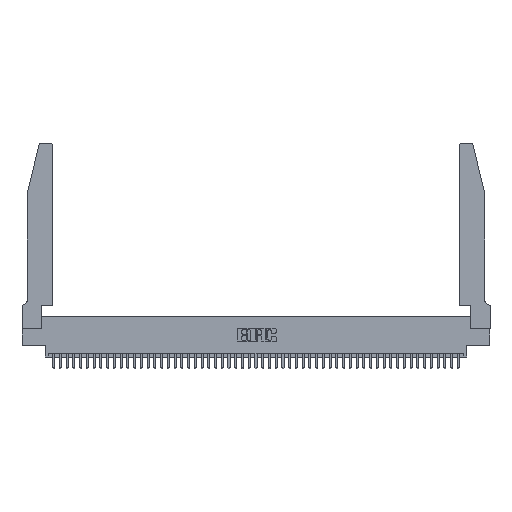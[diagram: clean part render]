
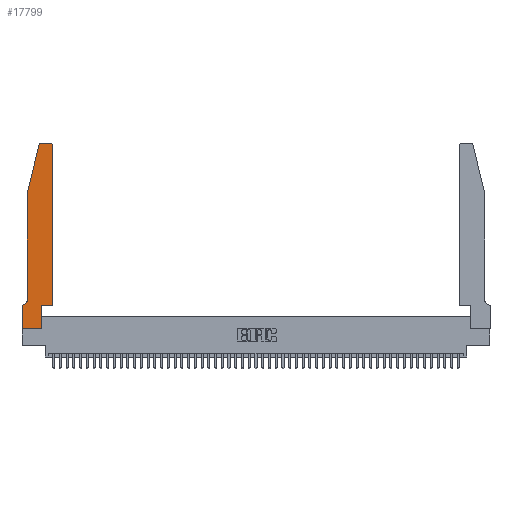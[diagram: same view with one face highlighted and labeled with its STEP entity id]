
A CAD part, top view. The second image highlights one B-rep face of the part: STEP entity #17799.
In plain terms, the highlighted planar face has unit normal (0, 0, 1).
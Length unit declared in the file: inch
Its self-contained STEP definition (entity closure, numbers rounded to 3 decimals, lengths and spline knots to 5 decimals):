
#931 = VERTEX_POINT ( 'NONE', #44905 ) ;
#1089 = LINE ( 'NONE', #2913, #20563 ) ;
#1990 = CARTESIAN_POINT ( 'NONE',  ( 0., 0., 0.37 ) ) ;
#2110 = EDGE_CURVE ( 'NONE', #21320, #24705, #28007, .T. ) ;
#2913 = CARTESIAN_POINT ( 'NONE',  ( 0., 0., 0.37 ) ) ;
#4332 = VECTOR ( 'NONE', #21773, 39.37008 ) ;
#4619 = CIRCLE ( 'NONE', #29182, 0.03 ) ;
#4855 = VECTOR ( 'NONE', #25329, 39.37008 ) ;
#6502 = CIRCLE ( 'NONE', #38145, 0.03 ) ;
#6902 = CARTESIAN_POINT ( 'NONE',  ( 0.4205, 2.72, 0.37 ) ) ;
#7082 = AXIS2_PLACEMENT_3D ( 'NONE', #7300, #34526, #11219 ) ;
#7300 = CARTESIAN_POINT ( 'NONE',  ( 0.0055, 0.42, 0.37 ) ) ;
#7564 = LINE ( 'NONE', #30500, #37380 ) ;
#8010 = VERTEX_POINT ( 'NONE', #41434 ) ;
#8220 = VERTEX_POINT ( 'NONE', #42438 ) ;
#9309 = FACE_OUTER_BOUND ( 'NONE', #49235, .T. ) ;
#10823 = DIRECTION ( 'NONE',  ( 1., 0., 0. ) ) ;
#11059 = VECTOR ( 'NONE', #26213, 39.37008 ) ;
#11179 = ORIENTED_EDGE ( 'NONE', *, *, #36745, .T. ) ;
#11219 = DIRECTION ( 'NONE',  ( -1., 0., 0. ) ) ;
#11917 = LINE ( 'NONE', #21364, #31407 ) ;
#11985 = EDGE_CURVE ( 'NONE', #36430, #46390, #40725, .T. ) ;
#12935 = CARTESIAN_POINT ( 'NONE',  ( 0., 0.35, 0.37 ) ) ;
#14453 = CARTESIAN_POINT ( 'NONE',  ( 0.4505, 0.35, 0.37 ) ) ;
#15032 = CARTESIAN_POINT ( 'NONE',  ( 0., 0., 0.37 ) ) ;
#15591 = VERTEX_POINT ( 'NONE', #47772 ) ;
#17471 = DIRECTION ( 'NONE',  ( 0., 1., 0. ) ) ;
#17622 = CARTESIAN_POINT ( 'NONE',  ( 0.0755, 2., 0.37 ) ) ;
#17799 = ADVANCED_FACE ( 'NONE', ( #9309 ), #46205, .T. ) ;
#17869 = CARTESIAN_POINT ( 'NONE',  ( 0.0755, 0.35, 0.37 ) ) ;
#18626 = VERTEX_POINT ( 'NONE', #50004 ) ;
#19388 = CARTESIAN_POINT ( 'NONE',  ( 0.284, 2.72, 0.37 ) ) ;
#20034 = VECTOR ( 'NONE', #36182, 39.37008 ) ;
#20265 = DIRECTION ( 'NONE',  ( 0., -1., 0. ) ) ;
#20518 = CARTESIAN_POINT ( 'NONE',  ( 0.4505, 0.35, 0.37 ) ) ;
#20535 = AXIS2_PLACEMENT_3D ( 'NONE', #49934, #50103, #49390 ) ;
#20563 = VECTOR ( 'NONE', #30157, 39.37008 ) ;
#21257 = ORIENTED_EDGE ( 'NONE', *, *, #28852, .T. ) ;
#21320 = VERTEX_POINT ( 'NONE', #12935 ) ;
#21356 = LINE ( 'NONE', #14453, #11059 ) ;
#21364 = CARTESIAN_POINT ( 'NONE',  ( 0.2865, 0.35, 0.37 ) ) ;
#21773 = DIRECTION ( 'NONE',  ( -1., 0., 0. ) ) ;
#22498 = ORIENTED_EDGE ( 'NONE', *, *, #32396, .T. ) ;
#22537 = LINE ( 'NONE', #40074, #41991 ) ;
#23283 = DIRECTION ( 'NONE',  ( 1., 0., 0. ) ) ;
#24360 = CARTESIAN_POINT ( 'NONE',  ( 0.0755, 2., 0.37 ) ) ;
#24492 = ORIENTED_EDGE ( 'NONE', *, *, #42632, .T. ) ;
#24635 = VERTEX_POINT ( 'NONE', #33761 ) ;
#24705 = VERTEX_POINT ( 'NONE', #15032 ) ;
#25047 = LINE ( 'NONE', #17869, #4332 ) ;
#25329 = DIRECTION ( 'NONE',  ( 0., -1., 0. ) ) ;
#25482 = ORIENTED_EDGE ( 'NONE', *, *, #11985, .T. ) ;
#26213 = DIRECTION ( 'NONE',  ( 0., 1., 0. ) ) ;
#26627 = ORIENTED_EDGE ( 'NONE', *, *, #48142, .T. ) ;
#27956 = VERTEX_POINT ( 'NONE', #17622 ) ;
#28007 = LINE ( 'NONE', #1990, #4855 ) ;
#28016 = CIRCLE ( 'NONE', #7082, 0.07 ) ;
#28852 = EDGE_CURVE ( 'NONE', #18626, #15591, #6502, .T. ) ;
#29182 = AXIS2_PLACEMENT_3D ( 'NONE', #6902, #34125, #10823 ) ;
#30157 = DIRECTION ( 'NONE',  ( 1., 0., 0. ) ) ;
#30500 = CARTESIAN_POINT ( 'NONE',  ( 0.0755, 2., 0.37 ) ) ;
#31108 = ORIENTED_EDGE ( 'NONE', *, *, #31866, .T. ) ;
#31407 = VECTOR ( 'NONE', #17471, 39.37008 ) ;
#31866 = EDGE_CURVE ( 'NONE', #8220, #21320, #25047, .T. ) ;
#32396 = EDGE_CURVE ( 'NONE', #24635, #18626, #22537, .T. ) ;
#33761 = CARTESIAN_POINT ( 'NONE',  ( 0.4205, 2.75, 0.37 ) ) ;
#34029 = VECTOR ( 'NONE', #20265, 39.37008 ) ;
#34125 = DIRECTION ( 'NONE',  ( 0., 0., 1. ) ) ;
#34526 = DIRECTION ( 'NONE',  ( 0., 0., -1. ) ) ;
#35197 = ORIENTED_EDGE ( 'NONE', *, *, #45778, .T. ) ;
#35243 = LINE ( 'NONE', #24360, #34029 ) ;
#36182 = DIRECTION ( 'NONE',  ( 1., 0., 0. ) ) ;
#36274 = CARTESIAN_POINT ( 'NONE',  ( 0.2865, 0.35, 0.37 ) ) ;
#36430 = VERTEX_POINT ( 'NONE', #36274 ) ;
#36745 = EDGE_CURVE ( 'NONE', #15591, #27956, #7564, .T. ) ;
#37380 = VECTOR ( 'NONE', #49810, 39.37008 ) ;
#38145 = AXIS2_PLACEMENT_3D ( 'NONE', #19388, #46567, #23283 ) ;
#39031 = EDGE_CURVE ( 'NONE', #8010, #8220, #28016, .T. ) ;
#39808 = ORIENTED_EDGE ( 'NONE', *, *, #2110, .T. ) ;
#40074 = CARTESIAN_POINT ( 'NONE',  ( 0.2605, 2.75, 0.37 ) ) ;
#40163 = CARTESIAN_POINT ( 'NONE',  ( 0.4505, 0.35, 0.37 ) ) ;
#40725 = LINE ( 'NONE', #20518, #20034 ) ;
#41086 = ORIENTED_EDGE ( 'NONE', *, *, #39031, .T. ) ;
#41434 = CARTESIAN_POINT ( 'NONE',  ( 0.0755, 0.42, 0.37 ) ) ;
#41991 = VECTOR ( 'NONE', #43945, 39.37008 ) ;
#42438 = CARTESIAN_POINT ( 'NONE',  ( 0.0055, 0.35, 0.37 ) ) ;
#42632 = EDGE_CURVE ( 'NONE', #46390, #931, #21356, .T. ) ;
#43945 = DIRECTION ( 'NONE',  ( -1., 0., 0. ) ) ;
#44342 = ORIENTED_EDGE ( 'NONE', *, *, #49696, .T. ) ;
#44905 = CARTESIAN_POINT ( 'NONE',  ( 0.4505, 2.72, 0.37 ) ) ;
#45778 = EDGE_CURVE ( 'NONE', #46461, #36430, #11917, .T. ) ;
#45904 = ORIENTED_EDGE ( 'NONE', *, *, #48452, .T. ) ;
#46205 = PLANE ( 'NONE',  #20535 ) ;
#46390 = VERTEX_POINT ( 'NONE', #40163 ) ;
#46461 = VERTEX_POINT ( 'NONE', #48465 ) ;
#46567 = DIRECTION ( 'NONE',  ( 0., 0., 1. ) ) ;
#47772 = CARTESIAN_POINT ( 'NONE',  ( 0.25487, 2.72718, 0.37 ) ) ;
#48142 = EDGE_CURVE ( 'NONE', #27956, #8010, #35243, .T. ) ;
#48452 = EDGE_CURVE ( 'NONE', #24705, #46461, #1089, .T. ) ;
#48465 = CARTESIAN_POINT ( 'NONE',  ( 0.2865, 0., 0.37 ) ) ;
#49235 = EDGE_LOOP ( 'NONE', ( #22498, #21257, #11179, #26627, #41086, #31108, #39808, #45904, #35197, #25482, #24492, #44342 ) ) ;
#49390 = DIRECTION ( 'NONE',  ( 1., 0., 0. ) ) ;
#49696 = EDGE_CURVE ( 'NONE', #931, #24635, #4619, .T. ) ;
#49810 = DIRECTION ( 'NONE',  ( -0.239, -0.971, 0. ) ) ;
#49934 = CARTESIAN_POINT ( 'NONE',  ( 0., 0.35, 0.37 ) ) ;
#50004 = CARTESIAN_POINT ( 'NONE',  ( 0.284, 2.75, 0.37 ) ) ;
#50103 = DIRECTION ( 'NONE',  ( 0., 0., 1. ) ) ;
